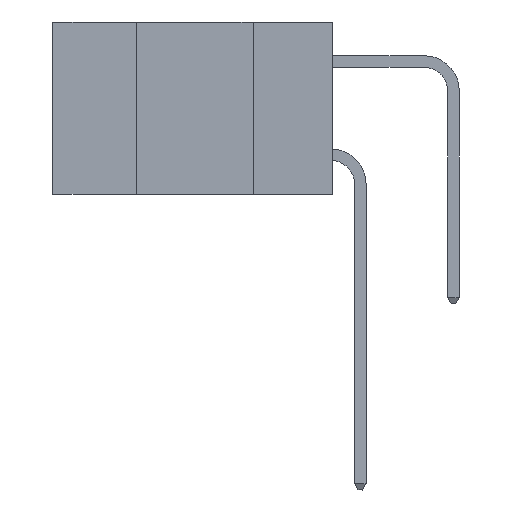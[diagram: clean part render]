
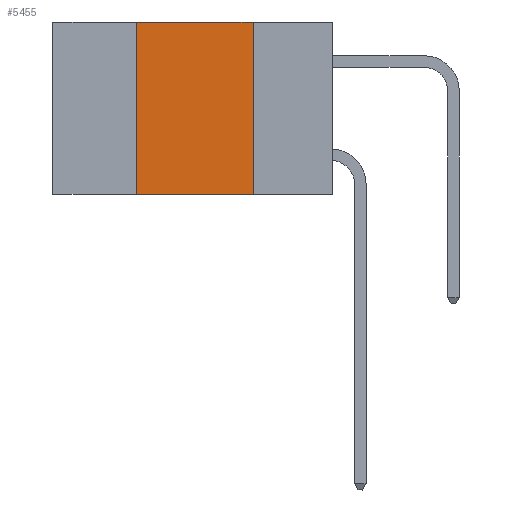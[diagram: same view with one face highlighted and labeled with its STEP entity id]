
A CAD part, left-side view. The second image highlights one B-rep face of the part: STEP entity #5455.
In plain terms, the highlighted planar face has unit normal (-1, 0, 0).
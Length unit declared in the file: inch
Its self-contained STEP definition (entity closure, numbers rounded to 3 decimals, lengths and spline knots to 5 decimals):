
#1464 = PLANE ( 'NONE',  #3951 ) ;
#2733 = CARTESIAN_POINT ( 'NONE',  ( 0., 0.42, 0. ) ) ;
#3344 = EDGE_LOOP ( 'NONE', ( #16772, #3762, #12389, #18179 ) ) ;
#3704 = VECTOR ( 'NONE', #8737, 39.37008 ) ;
#3762 = ORIENTED_EDGE ( 'NONE', *, *, #5430, .F. ) ;
#3856 = VERTEX_POINT ( 'NONE', #23887 ) ;
#3946 = LINE ( 'NONE', #18604, #31686 ) ;
#3951 = AXIS2_PLACEMENT_3D ( 'NONE', #6748, #3960, #13868 ) ;
#3960 = DIRECTION ( 'NONE',  ( 1., 0., 0. ) ) ;
#5157 = LINE ( 'NONE', #2733, #23178 ) ;
#5430 = EDGE_CURVE ( 'NONE', #8123, #25839, #5836, .T. ) ;
#5455 = ADVANCED_FACE ( 'NONE', ( #26637 ), #1464, .F. ) ;
#5836 = LINE ( 'NONE', #6548, #20869 ) ;
#6548 = CARTESIAN_POINT ( 'NONE',  ( 0., 0.6, 0. ) ) ;
#6748 = CARTESIAN_POINT ( 'NONE',  ( 0., 0.6, 0. ) ) ;
#8033 = EDGE_CURVE ( 'NONE', #25839, #3856, #8661, .T. ) ;
#8123 = VERTEX_POINT ( 'NONE', #29122 ) ;
#8661 = LINE ( 'NONE', #21153, #3704 ) ;
#8737 = DIRECTION ( 'NONE',  ( 0., 0., -1. ) ) ;
#10012 = EDGE_CURVE ( 'NONE', #18881, #3856, #3946, .T. ) ;
#10822 = DIRECTION ( 'NONE',  ( 0., 0., 1. ) ) ;
#12389 = ORIENTED_EDGE ( 'NONE', *, *, #17202, .F. ) ;
#13868 = DIRECTION ( 'NONE',  ( 0., 0., -1. ) ) ;
#14432 = CARTESIAN_POINT ( 'NONE',  ( 0., 0.17, 0. ) ) ;
#16413 = DIRECTION ( 'NONE',  ( 0., -1., 0. ) ) ;
#16772 = ORIENTED_EDGE ( 'NONE', *, *, #8033, .F. ) ;
#17202 = EDGE_CURVE ( 'NONE', #18881, #8123, #5157, .T. ) ;
#17437 = CARTESIAN_POINT ( 'NONE',  ( 0., 0.42, -0.37 ) ) ;
#18179 = ORIENTED_EDGE ( 'NONE', *, *, #10012, .T. ) ;
#18604 = CARTESIAN_POINT ( 'NONE',  ( 0., 0.6, -0.37 ) ) ;
#18881 = VERTEX_POINT ( 'NONE', #17437 ) ;
#20869 = VECTOR ( 'NONE', #16413, 39.37008 ) ;
#21153 = CARTESIAN_POINT ( 'NONE',  ( 0., 0.17, 0. ) ) ;
#23178 = VECTOR ( 'NONE', #10822, 39.37008 ) ;
#23887 = CARTESIAN_POINT ( 'NONE',  ( 0., 0.17, -0.37 ) ) ;
#25839 = VERTEX_POINT ( 'NONE', #14432 ) ;
#26637 = FACE_OUTER_BOUND ( 'NONE', #3344, .T. ) ;
#29122 = CARTESIAN_POINT ( 'NONE',  ( 0., 0.42, 0. ) ) ;
#31091 = DIRECTION ( 'NONE',  ( 0., -1., 0. ) ) ;
#31686 = VECTOR ( 'NONE', #31091, 39.37008 ) ;
